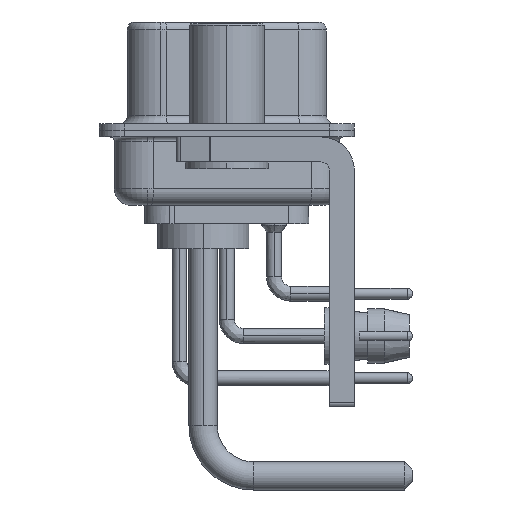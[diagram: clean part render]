
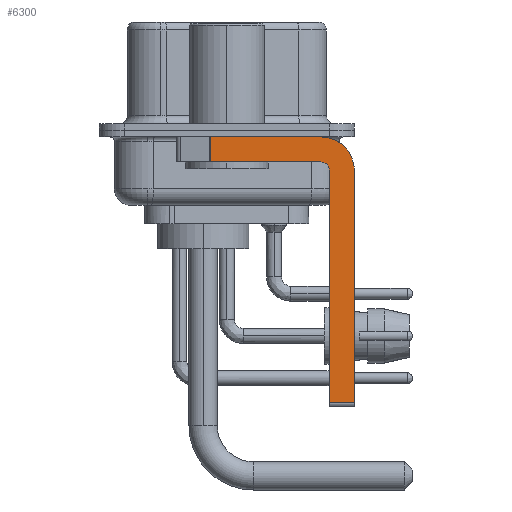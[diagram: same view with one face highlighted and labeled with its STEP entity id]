
A CAD part, left-side view. The second image highlights one B-rep face of the part: STEP entity #6300.
In plain terms, the highlighted planar face has unit normal (-1, 0, 0).
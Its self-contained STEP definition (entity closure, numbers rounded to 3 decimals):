
#71 = CIRCLE ( 'NONE', #23902, 2. ) ;
#1652 = VECTOR ( 'NONE', #22261, 1000. ) ;
#1950 = DIRECTION ( 'NONE',  ( -1., 0., 0. ) ) ;
#2364 = ORIENTED_EDGE ( 'NONE', *, *, #5638, .T. ) ;
#2576 = CARTESIAN_POINT ( 'NONE',  ( -2.9, -6.15, -2.4 ) ) ;
#3732 = LINE ( 'NONE', #20590, #6438 ) ;
#3867 = DIRECTION ( 'NONE',  ( 0., 0., -1. ) ) ;
#4543 = CARTESIAN_POINT ( 'NONE',  ( -2.9, -5.65, -1.9 ) ) ;
#5620 = CARTESIAN_POINT ( 'NONE',  ( -2.9, -6.15, -16.35 ) ) ;
#5638 = EDGE_CURVE ( 'NONE', #29816, #29180, #15374, .T. ) ;
#5950 = LINE ( 'NONE', #22814, #7149 ) ;
#6300 = ADVANCED_FACE ( 'NONE', ( #13729 ), #25931, .F. ) ;
#6399 = EDGE_CURVE ( 'NONE', #15985, #29180, #3732, .T. ) ;
#6438 = VECTOR ( 'NONE', #29545, 1000. ) ;
#7149 = VECTOR ( 'NONE', #11313, 1000. ) ;
#7906 = CARTESIAN_POINT ( 'NONE',  ( -2.9, 3., -0.4 ) ) ;
#8296 = CARTESIAN_POINT ( 'NONE',  ( -2.9, -5.65, -0.4 ) ) ;
#8734 = DIRECTION ( 'NONE',  ( 0., -1., 0. ) ) ;
#8892 = ORIENTED_EDGE ( 'NONE', *, *, #20430, .F. ) ;
#10828 = DIRECTION ( 'NONE',  ( 0., 0., -1. ) ) ;
#11209 = EDGE_LOOP ( 'NONE', ( #34484, #2364, #17081, #8892, #21950, #17651, #32997, #12345 ) ) ;
#11313 = DIRECTION ( 'NONE',  ( 0., 0., -1. ) ) ;
#12345 = ORIENTED_EDGE ( 'NONE', *, *, #29998, .F. ) ;
#12500 = VECTOR ( 'NONE', #3867, 1000. ) ;
#12665 = CARTESIAN_POINT ( 'NONE',  ( -2.9, -5.65, -2.4 ) ) ;
#13729 = FACE_OUTER_BOUND ( 'NONE', #11209, .T. ) ;
#13823 = CARTESIAN_POINT ( 'NONE',  ( -2.9, -5.65, -2.4 ) ) ;
#15061 = EDGE_CURVE ( 'NONE', #29816, #20179, #34443, .T. ) ;
#15374 = LINE ( 'NONE', #27013, #12500 ) ;
#15878 = EDGE_CURVE ( 'NONE', #34098, #24001, #32646, .T. ) ;
#15985 = VERTEX_POINT ( 'NONE', #4543 ) ;
#16007 = CIRCLE ( 'NONE', #35480, 0.5 ) ;
#16534 = EDGE_CURVE ( 'NONE', #21369, #21845, #5950, .T. ) ;
#17081 = ORIENTED_EDGE ( 'NONE', *, *, #6399, .F. ) ;
#17651 = ORIENTED_EDGE ( 'NONE', *, *, #34853, .T. ) ;
#17669 = CARTESIAN_POINT ( 'NONE',  ( -2.9, 0.978, -0.4 ) ) ;
#18037 = DIRECTION ( 'NONE',  ( 1., 0., 0. ) ) ;
#18145 = CARTESIAN_POINT ( 'NONE',  ( -2.9, -6.15, -16.6 ) ) ;
#19331 = CARTESIAN_POINT ( 'NONE',  ( -2.9, -7.65, -16.35 ) ) ;
#19751 = DIRECTION ( 'NONE',  ( 0., 0., 1. ) ) ;
#20006 = VECTOR ( 'NONE', #8734, 1000. ) ;
#20179 = VERTEX_POINT ( 'NONE', #8296 ) ;
#20430 = EDGE_CURVE ( 'NONE', #24001, #15985, #16007, .T. ) ;
#20590 = CARTESIAN_POINT ( 'NONE',  ( -2.9, -5.65, -1.9 ) ) ;
#21369 = VERTEX_POINT ( 'NONE', #27966 ) ;
#21845 = VERTEX_POINT ( 'NONE', #19331 ) ;
#21950 = ORIENTED_EDGE ( 'NONE', *, *, #15878, .F. ) ;
#22184 = CARTESIAN_POINT ( 'NONE',  ( -2.9, 0.978, -1.9 ) ) ;
#22261 = DIRECTION ( 'NONE',  ( 0., -1., 0. ) ) ;
#22814 = CARTESIAN_POINT ( 'NONE',  ( -2.9, -7.65, -2.4 ) ) ;
#23902 = AXIS2_PLACEMENT_3D ( 'NONE', #12665, #18037, #33288 ) ;
#24001 = VERTEX_POINT ( 'NONE', #2576 ) ;
#24076 = DIRECTION ( 'NONE',  ( 0., 0., 1. ) ) ;
#25931 = PLANE ( 'NONE',  #30232 ) ;
#25948 = LINE ( 'NONE', #26514, #20006 ) ;
#26514 = CARTESIAN_POINT ( 'NONE',  ( -2.9, -5.65, -16.35 ) ) ;
#27013 = CARTESIAN_POINT ( 'NONE',  ( -2.9, 0.978, -1.9 ) ) ;
#27966 = CARTESIAN_POINT ( 'NONE',  ( -2.9, -7.65, -2.4 ) ) ;
#29180 = VERTEX_POINT ( 'NONE', #22184 ) ;
#29545 = DIRECTION ( 'NONE',  ( 0., 1., 0. ) ) ;
#29816 = VERTEX_POINT ( 'NONE', #17669 ) ;
#29998 = EDGE_CURVE ( 'NONE', #20179, #21369, #71, .T. ) ;
#30232 = AXIS2_PLACEMENT_3D ( 'NONE', #37000, #37561, #10828 ) ;
#32127 = VECTOR ( 'NONE', #24076, 1000. ) ;
#32646 = LINE ( 'NONE', #18145, #32127 ) ;
#32997 = ORIENTED_EDGE ( 'NONE', *, *, #16534, .F. ) ;
#33288 = DIRECTION ( 'NONE',  ( 0., 0., -1. ) ) ;
#34098 = VERTEX_POINT ( 'NONE', #5620 ) ;
#34443 = LINE ( 'NONE', #7906, #1652 ) ;
#34484 = ORIENTED_EDGE ( 'NONE', *, *, #15061, .F. ) ;
#34853 = EDGE_CURVE ( 'NONE', #34098, #21845, #25948, .T. ) ;
#35480 = AXIS2_PLACEMENT_3D ( 'NONE', #13823, #1950, #19751 ) ;
#37000 = CARTESIAN_POINT ( 'NONE',  ( -2.9, -5.65, -2.4 ) ) ;
#37561 = DIRECTION ( 'NONE',  ( 1., 0., 0. ) ) ;
